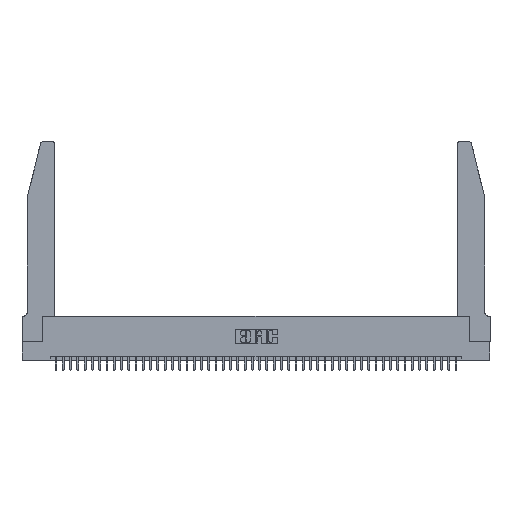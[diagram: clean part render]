
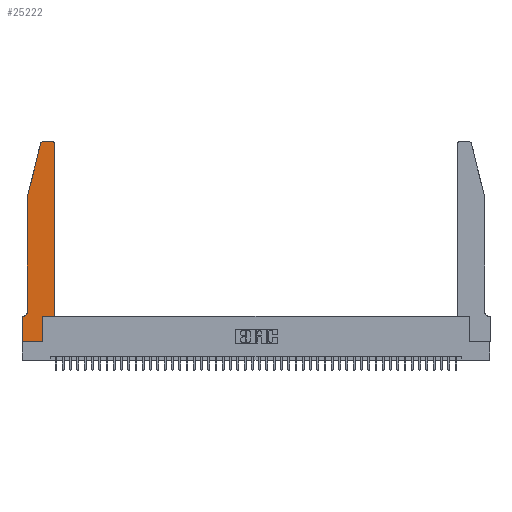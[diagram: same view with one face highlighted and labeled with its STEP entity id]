
A CAD part, top view. The second image highlights one B-rep face of the part: STEP entity #25222.
In plain terms, the highlighted planar face has unit normal (0, 0, 1).
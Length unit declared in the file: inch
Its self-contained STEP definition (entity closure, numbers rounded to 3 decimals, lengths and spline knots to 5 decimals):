
#369 = AXIS2_PLACEMENT_3D ( 'NONE', #18532, #43582, #22113 ) ;
#634 = ORIENTED_EDGE ( 'NONE', *, *, #14696, .T. ) ;
#1466 = VERTEX_POINT ( 'NONE', #4044 ) ;
#1586 = CIRCLE ( 'NONE', #40108, 0.03 ) ;
#2123 = VERTEX_POINT ( 'NONE', #25100 ) ;
#2332 = DIRECTION ( 'NONE',  ( 0., 0., 1. ) ) ;
#2714 = EDGE_CURVE ( 'NONE', #18753, #8888, #33119, .T. ) ;
#2946 = ORIENTED_EDGE ( 'NONE', *, *, #16140, .T. ) ;
#3390 = VERTEX_POINT ( 'NONE', #35993 ) ;
#3657 = CARTESIAN_POINT ( 'NONE',  ( 0.4505, 0.35, 0.37 ) ) ;
#4044 = CARTESIAN_POINT ( 'NONE',  ( 0.4505, 2.72, 0.37 ) ) ;
#4267 = DIRECTION ( 'NONE',  ( 0., 0., 1. ) ) ;
#4782 = CARTESIAN_POINT ( 'NONE',  ( 0.4205, 2.75, 0.37 ) ) ;
#5230 = CARTESIAN_POINT ( 'NONE',  ( 0., 0.35, 0.37 ) ) ;
#5429 = VECTOR ( 'NONE', #25213, 39.37008 ) ;
#5825 = ORIENTED_EDGE ( 'NONE', *, *, #29869, .T. ) ;
#7007 = EDGE_CURVE ( 'NONE', #7358, #1466, #40681, .T. ) ;
#7053 = VERTEX_POINT ( 'NONE', #16495 ) ;
#7235 = CARTESIAN_POINT ( 'NONE',  ( 0., 0., 0.37 ) ) ;
#7276 = VERTEX_POINT ( 'NONE', #14256 ) ;
#7358 = VERTEX_POINT ( 'NONE', #3657 ) ;
#7740 = VERTEX_POINT ( 'NONE', #34487 ) ;
#7972 = EDGE_CURVE ( 'NONE', #7276, #8109, #40590, .T. ) ;
#8089 = CARTESIAN_POINT ( 'NONE',  ( 0.2605, 2.75, 0.37 ) ) ;
#8109 = VERTEX_POINT ( 'NONE', #22619 ) ;
#8188 = EDGE_LOOP ( 'NONE', ( #25670, #8693, #18389, #30126, #41941, #23978, #5825, #36927, #46452, #634, #40287, #2946 ) ) ;
#8306 = DIRECTION ( 'NONE',  ( 0., 0., -1. ) ) ;
#8693 = ORIENTED_EDGE ( 'NONE', *, *, #23505, .T. ) ;
#8888 = VERTEX_POINT ( 'NONE', #5230 ) ;
#9459 = CARTESIAN_POINT ( 'NONE',  ( 0.0755, 2., 0.37 ) ) ;
#11082 = DIRECTION ( 'NONE',  ( 0., -1., 0. ) ) ;
#11708 = AXIS2_PLACEMENT_3D ( 'NONE', #24121, #2332, #27753 ) ;
#11895 = EDGE_CURVE ( 'NONE', #8109, #38074, #15867, .T. ) ;
#14024 = VECTOR ( 'NONE', #39803, 39.37008 ) ;
#14256 = CARTESIAN_POINT ( 'NONE',  ( 0., 0., 0.37 ) ) ;
#14696 = EDGE_CURVE ( 'NONE', #38074, #7358, #26732, .T. ) ;
#15867 = LINE ( 'NONE', #30240, #43369 ) ;
#15980 = DIRECTION ( 'NONE',  ( 0., 1., 0. ) ) ;
#16140 = EDGE_CURVE ( 'NONE', #1466, #40687, #1586, .T. ) ;
#16354 = LINE ( 'NONE', #9459, #35480 ) ;
#16495 = CARTESIAN_POINT ( 'NONE',  ( 0.25487, 2.72718, 0.37 ) ) ;
#17175 = VECTOR ( 'NONE', #44131, 39.37008 ) ;
#17545 = EDGE_CURVE ( 'NONE', #7053, #2123, #16354, .T. ) ;
#18014 = CARTESIAN_POINT ( 'NONE',  ( 0.0755, 2., 0.37 ) ) ;
#18389 = ORIENTED_EDGE ( 'NONE', *, *, #17545, .T. ) ;
#18471 = CARTESIAN_POINT ( 'NONE',  ( 0.0755, 0.35, 0.37 ) ) ;
#18532 = CARTESIAN_POINT ( 'NONE',  ( 0., 0.35, 0.37 ) ) ;
#18753 = VERTEX_POINT ( 'NONE', #22650 ) ;
#21124 = CARTESIAN_POINT ( 'NONE',  ( 0.4505, 0.35, 0.37 ) ) ;
#21456 = DIRECTION ( 'NONE',  ( 1., 0., 0. ) ) ;
#22035 = CIRCLE ( 'NONE', #39989, 0.07 ) ;
#22113 = DIRECTION ( 'NONE',  ( 1., 0., 0. ) ) ;
#22326 = EDGE_CURVE ( 'NONE', #7740, #18753, #22035, .T. ) ;
#22343 = VECTOR ( 'NONE', #11082, 39.37008 ) ;
#22619 = CARTESIAN_POINT ( 'NONE',  ( 0.2865, 0., 0.37 ) ) ;
#22650 = CARTESIAN_POINT ( 'NONE',  ( 0.0055, 0.35, 0.37 ) ) ;
#23505 = EDGE_CURVE ( 'NONE', #3390, #7053, #32007, .T. ) ;
#23978 = ORIENTED_EDGE ( 'NONE', *, *, #2714, .T. ) ;
#24000 = DIRECTION ( 'NONE',  ( -0.239, -0.971, 0. ) ) ;
#24121 = CARTESIAN_POINT ( 'NONE',  ( 0.284, 2.72, 0.37 ) ) ;
#24728 = DIRECTION ( 'NONE',  ( 1., 0., 0. ) ) ;
#25100 = CARTESIAN_POINT ( 'NONE',  ( 0.0755, 2., 0.37 ) ) ;
#25213 = DIRECTION ( 'NONE',  ( 0., -1., 0. ) ) ;
#25222 = ADVANCED_FACE ( 'NONE', ( #25708 ), #40012, .T. ) ;
#25670 = ORIENTED_EDGE ( 'NONE', *, *, #31113, .T. ) ;
#25708 = FACE_OUTER_BOUND ( 'NONE', #8188, .T. ) ;
#25873 = LINE ( 'NONE', #18014, #5429 ) ;
#26044 = CARTESIAN_POINT ( 'NONE',  ( 0.4205, 2.72, 0.37 ) ) ;
#26732 = LINE ( 'NONE', #21124, #36274 ) ;
#27753 = DIRECTION ( 'NONE',  ( 1., 0., 0. ) ) ;
#28479 = EDGE_CURVE ( 'NONE', #2123, #7740, #25873, .T. ) ;
#29616 = DIRECTION ( 'NONE',  ( 1., 0., 0. ) ) ;
#29869 = EDGE_CURVE ( 'NONE', #8888, #7276, #42555, .T. ) ;
#29886 = VECTOR ( 'NONE', #21456, 39.37008 ) ;
#29900 = CARTESIAN_POINT ( 'NONE',  ( 0.0055, 0.42, 0.37 ) ) ;
#30126 = ORIENTED_EDGE ( 'NONE', *, *, #28479, .T. ) ;
#30240 = CARTESIAN_POINT ( 'NONE',  ( 0.2865, 0.35, 0.37 ) ) ;
#31099 = VECTOR ( 'NONE', #34387, 39.37008 ) ;
#31113 = EDGE_CURVE ( 'NONE', #40687, #3390, #36284, .T. ) ;
#32007 = CIRCLE ( 'NONE', #11708, 0.03 ) ;
#33119 = LINE ( 'NONE', #18471, #14024 ) ;
#33516 = DIRECTION ( 'NONE',  ( -1., 0., 0. ) ) ;
#34387 = DIRECTION ( 'NONE',  ( 0., 1., 0. ) ) ;
#34487 = CARTESIAN_POINT ( 'NONE',  ( 0.0755, 0.42, 0.37 ) ) ;
#35480 = VECTOR ( 'NONE', #24000, 39.37008 ) ;
#35745 = CARTESIAN_POINT ( 'NONE',  ( 0., 0., 0.37 ) ) ;
#35993 = CARTESIAN_POINT ( 'NONE',  ( 0.284, 2.75, 0.37 ) ) ;
#36274 = VECTOR ( 'NONE', #24728, 39.37008 ) ;
#36284 = LINE ( 'NONE', #8089, #17175 ) ;
#36927 = ORIENTED_EDGE ( 'NONE', *, *, #7972, .T. ) ;
#38074 = VERTEX_POINT ( 'NONE', #40697 ) ;
#39803 = DIRECTION ( 'NONE',  ( -1., 0., 0. ) ) ;
#39989 = AXIS2_PLACEMENT_3D ( 'NONE', #29900, #8306, #33516 ) ;
#40012 = PLANE ( 'NONE',  #369 ) ;
#40108 = AXIS2_PLACEMENT_3D ( 'NONE', #26044, #4267, #29616 ) ;
#40287 = ORIENTED_EDGE ( 'NONE', *, *, #7007, .T. ) ;
#40590 = LINE ( 'NONE', #35745, #29886 ) ;
#40681 = LINE ( 'NONE', #45039, #31099 ) ;
#40687 = VERTEX_POINT ( 'NONE', #4782 ) ;
#40697 = CARTESIAN_POINT ( 'NONE',  ( 0.2865, 0.35, 0.37 ) ) ;
#41941 = ORIENTED_EDGE ( 'NONE', *, *, #22326, .T. ) ;
#42555 = LINE ( 'NONE', #7235, #22343 ) ;
#43369 = VECTOR ( 'NONE', #15980, 39.37008 ) ;
#43582 = DIRECTION ( 'NONE',  ( 0., 0., 1. ) ) ;
#44131 = DIRECTION ( 'NONE',  ( -1., 0., 0. ) ) ;
#45039 = CARTESIAN_POINT ( 'NONE',  ( 0.4505, 0.35, 0.37 ) ) ;
#46452 = ORIENTED_EDGE ( 'NONE', *, *, #11895, .T. ) ;
